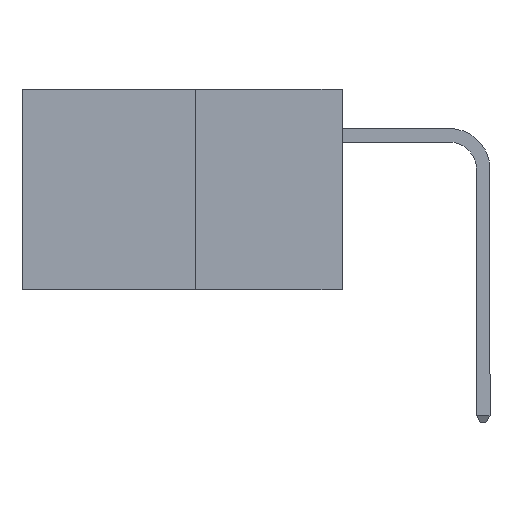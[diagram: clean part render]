
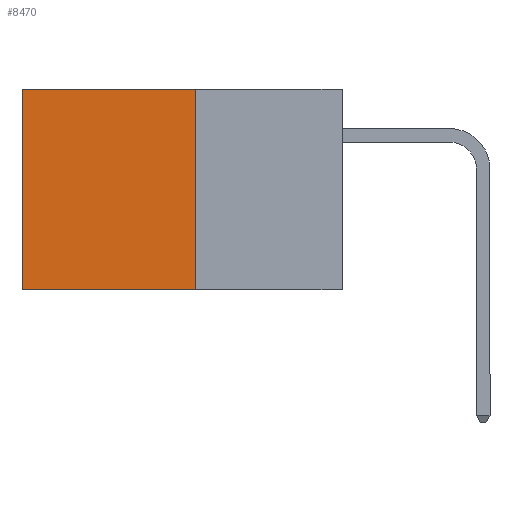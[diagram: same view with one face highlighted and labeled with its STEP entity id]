
A CAD part, left-side view. The second image highlights one B-rep face of the part: STEP entity #8470.
In plain terms, the highlighted planar face has unit normal (-1, 0, 0).
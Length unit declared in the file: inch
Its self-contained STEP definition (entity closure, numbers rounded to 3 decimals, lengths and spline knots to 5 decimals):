
#540 = ORIENTED_EDGE ( 'NONE', *, *, #2913, .F. ) ;
#551 = AXIS2_PLACEMENT_3D ( 'NONE', #9546, #12445, #6702 ) ;
#797 = VERTEX_POINT ( 'NONE', #11330 ) ;
#1693 = ORIENTED_EDGE ( 'NONE', *, *, #2032, .T. ) ;
#2032 = EDGE_CURVE ( 'NONE', #797, #6558, #6240, .T. ) ;
#2913 = EDGE_CURVE ( 'NONE', #4975, #9701, #9116, .T. ) ;
#3207 = ORIENTED_EDGE ( 'NONE', *, *, #5363, .T. ) ;
#3432 = ORIENTED_EDGE ( 'NONE', *, *, #4400, .F. ) ;
#4087 = FACE_OUTER_BOUND ( 'NONE', #9283, .T. ) ;
#4400 = EDGE_CURVE ( 'NONE', #9701, #6558, #10047, .T. ) ;
#4920 = CARTESIAN_POINT ( 'NONE',  ( 0.277, 0.27, -0.37 ) ) ;
#4975 = VERTEX_POINT ( 'NONE', #5834 ) ;
#5363 = EDGE_CURVE ( 'NONE', #4975, #797, #8501, .T. ) ;
#5834 = CARTESIAN_POINT ( 'NONE',  ( 0.277, 0.27, 0. ) ) ;
#5999 = CARTESIAN_POINT ( 'NONE',  ( 0.277, 0.59, -0.37 ) ) ;
#6212 = VECTOR ( 'NONE', #7394, 39.37008 ) ;
#6240 = LINE ( 'NONE', #5999, #12266 ) ;
#6558 = VERTEX_POINT ( 'NONE', #9045 ) ;
#6702 = DIRECTION ( 'NONE',  ( 0., 0., -1. ) ) ;
#7394 = DIRECTION ( 'NONE',  ( 0., 1., 0. ) ) ;
#7408 = CARTESIAN_POINT ( 'NONE',  ( 0.277, 0.27, 0. ) ) ;
#8470 = ADVANCED_FACE ( 'NONE', ( #4087 ), #11529, .F. ) ;
#8501 = LINE ( 'NONE', #7408, #6212 ) ;
#8564 = DIRECTION ( 'NONE',  ( 0., 1., 0. ) ) ;
#8612 = CARTESIAN_POINT ( 'NONE',  ( 0.277, 0.27, -0.37 ) ) ;
#8807 = VECTOR ( 'NONE', #9787, 39.37008 ) ;
#9045 = CARTESIAN_POINT ( 'NONE',  ( 0.277, 0.59, -0.37 ) ) ;
#9116 = LINE ( 'NONE', #9957, #8807 ) ;
#9179 = DIRECTION ( 'NONE',  ( 0., 0., -1. ) ) ;
#9283 = EDGE_LOOP ( 'NONE', ( #1693, #3432, #540, #3207 ) ) ;
#9546 = CARTESIAN_POINT ( 'NONE',  ( 0.277, 0.27, -0.37 ) ) ;
#9701 = VERTEX_POINT ( 'NONE', #4920 ) ;
#9787 = DIRECTION ( 'NONE',  ( 0., 0., -1. ) ) ;
#9957 = CARTESIAN_POINT ( 'NONE',  ( 0.277, 0.27, -0.37 ) ) ;
#10047 = LINE ( 'NONE', #8612, #12545 ) ;
#11330 = CARTESIAN_POINT ( 'NONE',  ( 0.277, 0.59, 0. ) ) ;
#11529 = PLANE ( 'NONE',  #551 ) ;
#12266 = VECTOR ( 'NONE', #9179, 39.37008 ) ;
#12445 = DIRECTION ( 'NONE',  ( 1., 0., 0. ) ) ;
#12545 = VECTOR ( 'NONE', #8564, 39.37008 ) ;
